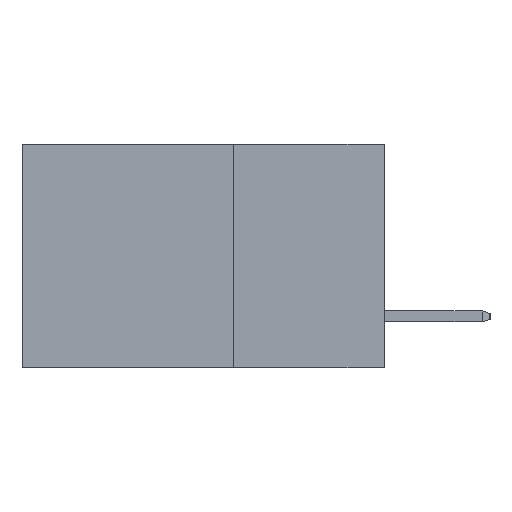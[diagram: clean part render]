
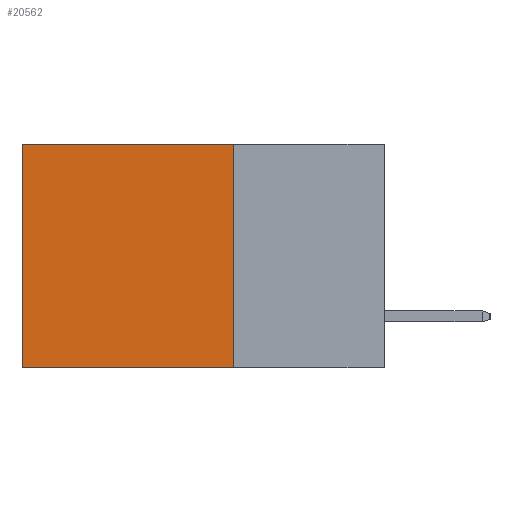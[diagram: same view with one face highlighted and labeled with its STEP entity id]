
A CAD part, left-side view. The second image highlights one B-rep face of the part: STEP entity #20562.
In plain terms, the highlighted planar face has unit normal (-1, 0, 0).
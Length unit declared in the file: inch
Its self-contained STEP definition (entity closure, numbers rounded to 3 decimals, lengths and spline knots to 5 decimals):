
#57 = LINE ( 'NONE', #13427, #20544 ) ;
#354 = LINE ( 'NONE', #22547, #14370 ) ;
#520 = CARTESIAN_POINT ( 'NONE',  ( 0.2615, 0.25, -0.37 ) ) ;
#789 = VECTOR ( 'NONE', #10899, 39.37008 ) ;
#1972 = EDGE_CURVE ( 'NONE', #23920, #11400, #354, .T. ) ;
#3983 = FACE_OUTER_BOUND ( 'NONE', #24344, .T. ) ;
#5139 = ORIENTED_EDGE ( 'NONE', *, *, #18161, .T. ) ;
#5481 = ORIENTED_EDGE ( 'NONE', *, *, #1972, .F. ) ;
#7050 = DIRECTION ( 'NONE',  ( 0., 0., -1. ) ) ;
#8368 = LINE ( 'NONE', #22404, #17666 ) ;
#8983 = PLANE ( 'NONE',  #23449 ) ;
#10643 = DIRECTION ( 'NONE',  ( 0., 0., -1. ) ) ;
#10899 = DIRECTION ( 'NONE',  ( 0., 0., -1. ) ) ;
#11400 = VERTEX_POINT ( 'NONE', #18616 ) ;
#12967 = CARTESIAN_POINT ( 'NONE',  ( 0.2615, 0.25, -0.37 ) ) ;
#13427 = CARTESIAN_POINT ( 'NONE',  ( 0.2615, 0.25, 0. ) ) ;
#14370 = VECTOR ( 'NONE', #22657, 39.37008 ) ;
#14653 = ORIENTED_EDGE ( 'NONE', *, *, #20436, .T. ) ;
#15314 = CARTESIAN_POINT ( 'NONE',  ( 0.2615, 0.6, 0. ) ) ;
#16039 = LINE ( 'NONE', #22656, #789 ) ;
#17360 = VERTEX_POINT ( 'NONE', #21121 ) ;
#17666 = VECTOR ( 'NONE', #10643, 39.37008 ) ;
#18161 = EDGE_CURVE ( 'NONE', #17360, #24107, #57, .T. ) ;
#18616 = CARTESIAN_POINT ( 'NONE',  ( 0.2615, 0.6, -0.37 ) ) ;
#18923 = DIRECTION ( 'NONE',  ( 1., 0., 0. ) ) ;
#19372 = DIRECTION ( 'NONE',  ( 0., 1., 0. ) ) ;
#20436 = EDGE_CURVE ( 'NONE', #24107, #11400, #8368, .T. ) ;
#20544 = VECTOR ( 'NONE', #19372, 39.37008 ) ;
#20562 = ADVANCED_FACE ( 'NONE', ( #3983 ), #8983, .F. ) ;
#21121 = CARTESIAN_POINT ( 'NONE',  ( 0.2615, 0.25, 0. ) ) ;
#22404 = CARTESIAN_POINT ( 'NONE',  ( 0.2615, 0.6, -0.37 ) ) ;
#22547 = CARTESIAN_POINT ( 'NONE',  ( 0.2615, 0.25, -0.37 ) ) ;
#22571 = EDGE_CURVE ( 'NONE', #17360, #23920, #16039, .T. ) ;
#22656 = CARTESIAN_POINT ( 'NONE',  ( 0.2615, 0.25, -0.37 ) ) ;
#22657 = DIRECTION ( 'NONE',  ( 0., 1., 0. ) ) ;
#22805 = ORIENTED_EDGE ( 'NONE', *, *, #22571, .F. ) ;
#23449 = AXIS2_PLACEMENT_3D ( 'NONE', #12967, #18923, #7050 ) ;
#23920 = VERTEX_POINT ( 'NONE', #520 ) ;
#24107 = VERTEX_POINT ( 'NONE', #15314 ) ;
#24344 = EDGE_LOOP ( 'NONE', ( #14653, #5481, #22805, #5139 ) ) ;
